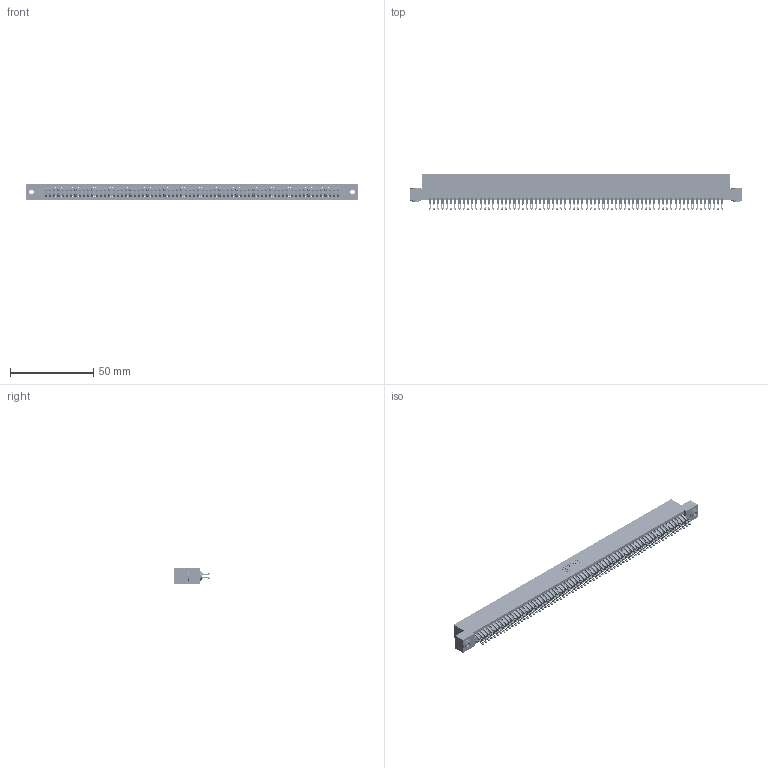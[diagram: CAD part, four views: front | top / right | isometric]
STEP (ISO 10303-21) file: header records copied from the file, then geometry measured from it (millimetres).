
FILE_DESCRIPTION (( 'STEP AP203' ), '1' );
FILE_NAME ('345-140-555-203.STEP', '2018-10-21T00:58:52', ( '' ), ( '' ), 'SwSTEP 2.0', 'SolidWorks 2016', '' );
FILE_SCHEMA (( 'CONFIG_CONTROL_DESIGN' ));
Length unit declared in the file: inch
Products named in the file (4): 345 Part_Flush Mounting Lugs - 0.156 Dia-TH; 345-250-002_345-250-002-102; 345-140-555-203; 345-292-001_555 Tail
Assembly tree (143 placements, depth 2):
  345-140-555-203
    345 Part_Flush Mounting Lugs - 0.156 Dia-TH
    345-292-001_555 Tail  x140
    345-250-002_345-250-002-102  x2
Bounding box: 199.01 x 21.13 x 9.4 mm (x, y, z)
Volume: 20017.3 mm3; surface area: 31748.5 mm2
Topology: 143 solids, 143 shells, 8004 faces, 25197 edges, 16794 vertices
Faces by surface type: plane 4430, cylinder 3566, cone 8
Entity records: 52130 total; most frequent: CARTESIAN_POINT 8721, ORIENTED_EDGE 8618, DIRECTION 7655, EDGE_CURVE 4309, LINE 3853, VECTOR 3853, VERTEX_POINT 2870, AXIS2_PLACEMENT_3D 1901
